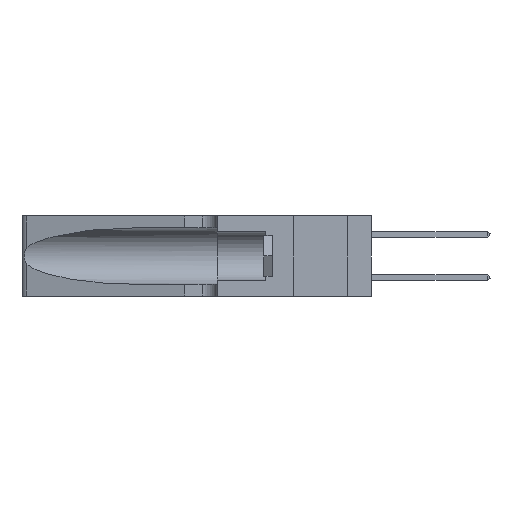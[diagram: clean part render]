
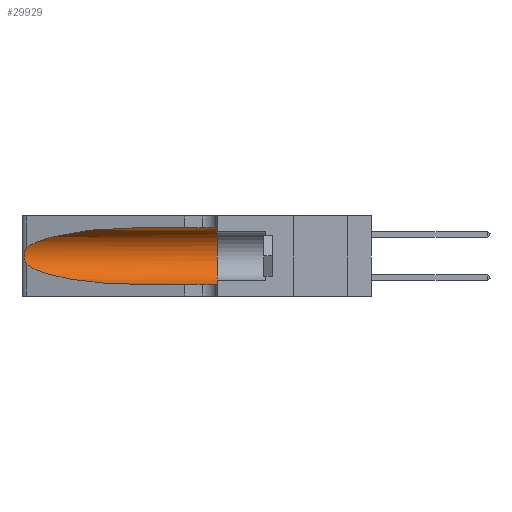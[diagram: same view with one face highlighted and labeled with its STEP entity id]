
A CAD part, left-side view. The second image highlights one B-rep face of the part: STEP entity #29929.
In plain terms, the highlighted cylindrical face has radius 3.308 mm (diameter 6.617 mm), a partial arc.
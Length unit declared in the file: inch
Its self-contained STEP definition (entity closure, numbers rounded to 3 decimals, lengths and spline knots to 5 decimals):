
#96 = CARTESIAN_POINT ( 'NONE',  ( 0.1305, 0.35, 0.185 ) ) ;
#502 = CARTESIAN_POINT ( 'NONE',  ( 0.26017, 1.23833, 0.17102 ) ) ;
#909 = VERTEX_POINT ( 'NONE', #11981 ) ;
#1683 = DIRECTION ( 'NONE',  ( 0., 0., -1. ) ) ;
#2154 = CARTESIAN_POINT ( 'NONE',  ( 0.2373, 1.15595, 0.08982 ) ) ;
#3098 = DIRECTION ( 'NONE',  ( 0., 0., 1. ) ) ;
#3446 = VERTEX_POINT ( 'NONE', #14436 ) ;
#3501 = CARTESIAN_POINT ( 'NONE',  ( 0.25789, 1.23486, 0.15765 ) ) ;
#4273 = CARTESIAN_POINT ( 'NONE',  ( 0.18966, 0.96281, 0.31525 ) ) ;
#4409 = ORIENTED_EDGE ( 'NONE', *, *, #8367, .F. ) ;
#5656 = AXIS2_PLACEMENT_3D ( 'NONE', #16542, #19547, #1683 ) ;
#6285 = EDGE_CURVE ( 'NONE', #18375, #30880, #20982, .T. ) ;
#6531 = CARTESIAN_POINT ( 'NONE',  ( 0.25555, 1.22993, 0.14849 ) ) ;
#7511 = EDGE_CURVE ( 'NONE', #30880, #8612, #8167, .T. ) ;
#7920 = CARTESIAN_POINT ( 'NONE',  ( 0.25487, 1.22718, 0.22369 ) ) ;
#8167 = LINE ( 'NONE', #11389, #25909 ) ;
#8367 = EDGE_CURVE ( 'NONE', #3446, #8612, #25839, .T. ) ;
#8612 = VERTEX_POINT ( 'NONE', #33972 ) ;
#10280 = CARTESIAN_POINT ( 'NONE',  ( 0.25487, 1.22718, 0.22369 ) ) ;
#10418 = VERTEX_POINT ( 'NONE', #7920 ) ;
#11168 = CARTESIAN_POINT ( 'NONE',  ( 0.18966, 0.96281, 0.05475 ) ) ;
#11389 = CARTESIAN_POINT ( 'NONE',  ( 0.1305, 1.61858, 0.05475 ) ) ;
#11981 = CARTESIAN_POINT ( 'NONE',  ( 0.1305, 0.72297, 0.31525 ) ) ;
#12360 = CARTESIAN_POINT ( 'NONE',  ( 0.25787, 1.23484, 0.2124 ) ) ;
#12846 = B_SPLINE_CURVE_WITH_KNOTS ( 'NONE', 3,
 ( #27261, #24261, #30219, #12360, #33209, #15355, #36165, #18343, #502, #21378, #3501, #24400, #6531, #27392 ),
 .UNSPECIFIED., .F., .F.,
 ( 4, 2, 2, 2, 2, 2, 4 ),
 ( 0., 0.00027, 0.00053, 0.00107, 0.0016, 0.00187, 0.00214 ),
 .UNSPECIFIED. ) ;
#14436 = CARTESIAN_POINT ( 'NONE',  ( 0.1305, 0.35, 0.31525 ) ) ;
#15355 = CARTESIAN_POINT ( 'NONE',  ( 0.26018, 1.23835, 0.19895 ) ) ;
#16542 = CARTESIAN_POINT ( 'NONE',  ( 0.1305, 1.61858, 0.185 ) ) ;
#17020 = ORIENTED_EDGE ( 'NONE', *, *, #30189, .T. ) ;
#17114 = CARTESIAN_POINT ( 'NONE',  ( 0.25487, 1.22718, 0.14631 ) ) ;
#17683 = CARTESIAN_POINT ( 'NONE',  ( 0.25487, 1.22718, 0.14631 ) ) ;
#18343 = CARTESIAN_POINT ( 'NONE',  ( 0.26075, 1.23896, 0.178 ) ) ;
#18375 = VERTEX_POINT ( 'NONE', #17683 ) ;
#18940 = DIRECTION ( 'NONE',  ( 0., -1., 0. ) ) ;
#19314 = ORIENTED_EDGE ( 'NONE', *, *, #7511, .T. ) ;
#19547 = DIRECTION ( 'NONE',  ( 0., -1., 0. ) ) ;
#19781 =( BOUNDED_CURVE ( )  B_SPLINE_CURVE ( 3, ( #22138, #4273, #28148, #10280 ),
 .UNSPECIFIED., .F., .T. ) 
 B_SPLINE_CURVE_WITH_KNOTS ( ( 4, 4 ),
 ( 1.5708, 2.84003 ),
 .UNSPECIFIED. ) 
 CURVE ( )  GEOMETRIC_REPRESENTATION_ITEM ( )  RATIONAL_B_SPLINE_CURVE ( ( 1., 0.87, 0.87, 1. ) ) 
 REPRESENTATION_ITEM ( '' )  );
#20977 = DIRECTION ( 'NONE',  ( 0., 1., 0. ) ) ;
#20982 =( BOUNDED_CURVE ( )  B_SPLINE_CURVE ( 3, ( #17114, #2154, #11168, #37935 ),
 .UNSPECIFIED., .F., .T. ) 
 B_SPLINE_CURVE_WITH_KNOTS ( ( 4, 4 ),
 ( 3.44316, 4.71239 ),
 .UNSPECIFIED. ) 
 CURVE ( )  GEOMETRIC_REPRESENTATION_ITEM ( )  RATIONAL_B_SPLINE_CURVE ( ( 1., 0.87, 0.87, 1. ) ) 
 REPRESENTATION_ITEM ( '' )  );
#21378 = CARTESIAN_POINT ( 'NONE',  ( 0.25856, 1.23593, 0.16098 ) ) ;
#21458 = CARTESIAN_POINT ( 'NONE',  ( 0.1305, 0.72297, 0.05475 ) ) ;
#22138 = CARTESIAN_POINT ( 'NONE',  ( 0.1305, 0.72297, 0.31525 ) ) ;
#22147 = ORIENTED_EDGE ( 'NONE', *, *, #32699, .F. ) ;
#23735 = VECTOR ( 'NONE', #18940, 39.37008 ) ;
#24069 = ORIENTED_EDGE ( 'NONE', *, *, #36290, .T. ) ;
#24261 = CARTESIAN_POINT ( 'NONE',  ( 0.25555, 1.22994, 0.2215 ) ) ;
#24400 = CARTESIAN_POINT ( 'NONE',  ( 0.25639, 1.23186, 0.15144 ) ) ;
#25839 = CIRCLE ( 'NONE', #34184, 0.13025 ) ;
#25909 = VECTOR ( 'NONE', #35185, 39.37008 ) ;
#26884 = ORIENTED_EDGE ( 'NONE', *, *, #6285, .T. ) ;
#27261 = CARTESIAN_POINT ( 'NONE',  ( 0.25487, 1.22718, 0.22369 ) ) ;
#27392 = CARTESIAN_POINT ( 'NONE',  ( 0.25487, 1.22718, 0.14631 ) ) ;
#28148 = CARTESIAN_POINT ( 'NONE',  ( 0.2373, 1.15595, 0.28018 ) ) ;
#29929 = ADVANCED_FACE ( 'NONE', ( #36788 ), #35862, .F. ) ;
#29982 = EDGE_LOOP ( 'NONE', ( #24069, #17020, #26884, #19314, #4409, #22147 ) ) ;
#30189 = EDGE_CURVE ( 'NONE', #10418, #18375, #12846, .T. ) ;
#30219 = CARTESIAN_POINT ( 'NONE',  ( 0.25639, 1.23184, 0.21858 ) ) ;
#30721 = LINE ( 'NONE', #36746, #23735 ) ;
#30880 = VERTEX_POINT ( 'NONE', #21458 ) ;
#32699 = EDGE_CURVE ( 'NONE', #909, #3446, #30721, .T. ) ;
#33209 = CARTESIAN_POINT ( 'NONE',  ( 0.25854, 1.2359, 0.20912 ) ) ;
#33972 = CARTESIAN_POINT ( 'NONE',  ( 0.1305, 0.35, 0.05475 ) ) ;
#34184 = AXIS2_PLACEMENT_3D ( 'NONE', #96, #20977, #3098 ) ;
#35185 = DIRECTION ( 'NONE',  ( 0., -1., 0. ) ) ;
#35862 = CYLINDRICAL_SURFACE ( 'NONE', #5656, 0.13025 ) ;
#36165 = CARTESIAN_POINT ( 'NONE',  ( 0.26075, 1.23896, 0.19203 ) ) ;
#36290 = EDGE_CURVE ( 'NONE', #909, #10418, #19781, .T. ) ;
#36746 = CARTESIAN_POINT ( 'NONE',  ( 0.1305, 1.61858, 0.31525 ) ) ;
#36788 = FACE_OUTER_BOUND ( 'NONE', #29982, .T. ) ;
#37935 = CARTESIAN_POINT ( 'NONE',  ( 0.1305, 0.72297, 0.05475 ) ) ;
